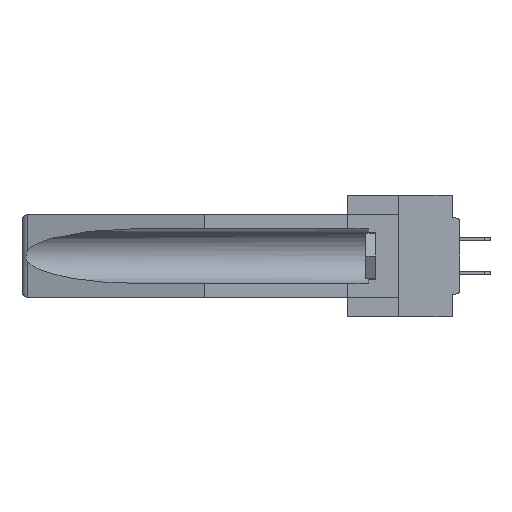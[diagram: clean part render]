
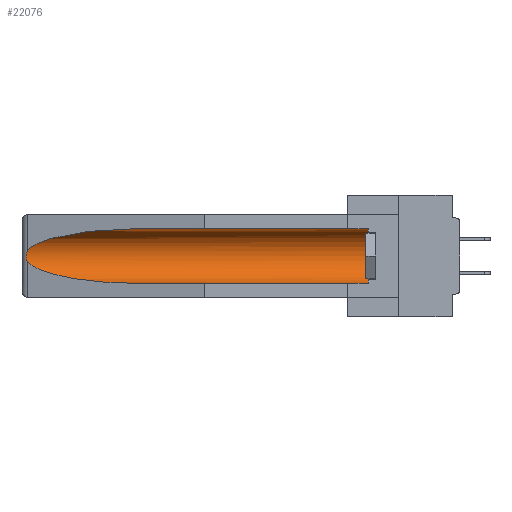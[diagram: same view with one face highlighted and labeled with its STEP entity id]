
A CAD part, left-side view. The second image highlights one B-rep face of the part: STEP entity #22076.
In plain terms, the highlighted cylindrical face has radius 2.857 mm (diameter 5.715 mm), a partial arc.
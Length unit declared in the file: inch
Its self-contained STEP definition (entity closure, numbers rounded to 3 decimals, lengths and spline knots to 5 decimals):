
#261 = CARTESIAN_POINT ( 'NONE',  ( 0.2673, 1.5327, -0.16383 ) ) ;
#477 = DIRECTION ( 'NONE',  ( 0., 0., 1. ) ) ;
#1191 = EDGE_CURVE ( 'NONE', #8287, #29350, #18271, .T. ) ;
#1553 = DIRECTION ( 'NONE',  ( 0., 1., 0. ) ) ;
#1906 = CYLINDRICAL_SURFACE ( 'NONE', #4686, 0.1125 ) ;
#2581 = VECTOR ( 'NONE', #31419, 39.37008 ) ;
#2783 = CARTESIAN_POINT ( 'NONE',  ( 0.26537, 1.52718, -0.14972 ) ) ;
#3278 = EDGE_CURVE ( 'NONE', #26897, #29350, #33648, .T. ) ;
#4251 = CARTESIAN_POINT ( 'NONE',  ( 0.155, 0.126, -0.1715 ) ) ;
#4686 = AXIS2_PLACEMENT_3D ( 'NONE', #19137, #5865, #477 ) ;
#5775 = CARTESIAN_POINT ( 'NONE',  ( 0.26537, 1.52718, -0.14972 ) ) ;
#5865 = DIRECTION ( 'NONE',  ( 0., 1., 0. ) ) ;
#5871 = LINE ( 'NONE', #21099, #2581 ) ;
#6681 = EDGE_LOOP ( 'NONE', ( #30616, #13603, #9948, #15802, #29697, #26227 ) ) ;
#6843 = EDGE_CURVE ( 'NONE', #8287, #15773, #15491, .T. ) ;
#7047 = CARTESIAN_POINT ( 'NONE',  ( 0.25451, 1.48313, -0.09465 ) ) ;
#8269 = CARTESIAN_POINT ( 'NONE',  ( 0.155, 1.07973, -0.284 ) ) ;
#8287 = VERTEX_POINT ( 'NONE', #11975 ) ;
#8763 = CARTESIAN_POINT ( 'NONE',  ( 0.26655, 1.53094, -0.18657 ) ) ;
#8972 = CARTESIAN_POINT ( 'NONE',  ( 0.155, 1.07973, -0.059 ) ) ;
#9255 = CARTESIAN_POINT ( 'NONE',  ( 0.26537, 1.52718, -0.14972 ) ) ;
#9948 = ORIENTED_EDGE ( 'NONE', *, *, #3278, .T. ) ;
#10777 = CARTESIAN_POINT ( 'NONE',  ( 0.2675, 1.53308, -0.17534 ) ) ;
#11446 = CARTESIAN_POINT ( 'NONE',  ( 0.155, 1.07973, -0.284 ) ) ;
#11547 = CARTESIAN_POINT ( 'NONE',  ( 0.26537, 1.52718, -0.19328 ) ) ;
#11863 = VERTEX_POINT ( 'NONE', #8972 ) ;
#11953 = CARTESIAN_POINT ( 'NONE',  ( 0.155, -0.30754, -0.284 ) ) ;
#11975 = CARTESIAN_POINT ( 'NONE',  ( 0.155, 0.126, -0.284 ) ) ;
#13603 = ORIENTED_EDGE ( 'NONE', *, *, #27464, .T. ) ;
#14019 = CARTESIAN_POINT ( 'NONE',  ( 0.21114, 1.30732, -0.284 ) ) ;
#14381 = EDGE_CURVE ( 'NONE', #11863, #25682, #33209, .T. ) ;
#15491 = CIRCLE ( 'NONE', #28461, 0.1125 ) ;
#15773 = VERTEX_POINT ( 'NONE', #25791 ) ;
#15802 = ORIENTED_EDGE ( 'NONE', *, *, #1191, .F. ) ;
#16107 = CARTESIAN_POINT ( 'NONE',  ( 0.2675, 1.53308, -0.16763 ) ) ;
#18271 = LINE ( 'NONE', #11953, #32357 ) ;
#19137 = CARTESIAN_POINT ( 'NONE',  ( 0.155, -0.30754, -0.1715 ) ) ;
#21099 = CARTESIAN_POINT ( 'NONE',  ( 0.155, -0.30754, -0.059 ) ) ;
#22053 = CARTESIAN_POINT ( 'NONE',  ( 0.26537, 1.52718, -0.19328 ) ) ;
#22076 = ADVANCED_FACE ( 'NONE', ( #30542 ), #1906, .F. ) ;
#22987 = CARTESIAN_POINT ( 'NONE',  ( 0.21114, 1.30732, -0.059 ) ) ;
#23305 = DIRECTION ( 'NONE',  ( 0., -1., 0. ) ) ;
#23872 = B_SPLINE_CURVE_WITH_KNOTS ( 'NONE', 3,
 ( #5775, #24029, #26701, #261, #16107, #10777, #29366, #8763, #27479, #11547 ),
 .UNSPECIFIED., .F., .F.,
 ( 4, 2, 2, 2, 4 ),
 ( 0., 0.00029, 0.00058, 0.00087, 0.00117 ),
 .UNSPECIFIED. ) ;
#24029 = CARTESIAN_POINT ( 'NONE',  ( 0.26597, 1.52961, -0.15275 ) ) ;
#24496 = CARTESIAN_POINT ( 'NONE',  ( 0.26537, 1.52718, -0.19328 ) ) ;
#24629 = EDGE_CURVE ( 'NONE', #15773, #11863, #5871, .T. ) ;
#25682 = VERTEX_POINT ( 'NONE', #2783 ) ;
#25791 = CARTESIAN_POINT ( 'NONE',  ( 0.155, 0.126, -0.059 ) ) ;
#26227 = ORIENTED_EDGE ( 'NONE', *, *, #24629, .T. ) ;
#26701 = CARTESIAN_POINT ( 'NONE',  ( 0.26654, 1.53092, -0.15636 ) ) ;
#26897 = VERTEX_POINT ( 'NONE', #24496 ) ;
#27464 = EDGE_CURVE ( 'NONE', #25682, #26897, #23872, .T. ) ;
#27479 = CARTESIAN_POINT ( 'NONE',  ( 0.26597, 1.5296, -0.19026 ) ) ;
#28461 = AXIS2_PLACEMENT_3D ( 'NONE', #4251, #23305, #28992 ) ;
#28992 = DIRECTION ( 'NONE',  ( 0., 0., 1. ) ) ;
#29350 = VERTEX_POINT ( 'NONE', #8269 ) ;
#29366 = CARTESIAN_POINT ( 'NONE',  ( 0.2673, 1.53269, -0.17917 ) ) ;
#29697 = ORIENTED_EDGE ( 'NONE', *, *, #6843, .T. ) ;
#30542 = FACE_OUTER_BOUND ( 'NONE', #6681, .T. ) ;
#30616 = ORIENTED_EDGE ( 'NONE', *, *, #14381, .T. ) ;
#31419 = DIRECTION ( 'NONE',  ( 0., 1., 0. ) ) ;
#32254 = CARTESIAN_POINT ( 'NONE',  ( 0.25451, 1.48313, -0.24835 ) ) ;
#32357 = VECTOR ( 'NONE', #1553, 39.37008 ) ;
#33209 =( BOUNDED_CURVE ( )  B_SPLINE_CURVE ( 3, ( #33545, #22987, #7047, #9255 ),
 .UNSPECIFIED., .F., .F. ) 
 B_SPLINE_CURVE_WITH_KNOTS ( ( 4, 4 ),
 ( 4.71239, 6.08839 ),
 .UNSPECIFIED. ) 
 CURVE ( )  GEOMETRIC_REPRESENTATION_ITEM ( )  RATIONAL_B_SPLINE_CURVE ( ( 1., 0.848, 0.848, 1. ) ) 
 REPRESENTATION_ITEM ( '' )  );
#33545 = CARTESIAN_POINT ( 'NONE',  ( 0.155, 1.07973, -0.059 ) ) ;
#33648 =( BOUNDED_CURVE ( )  B_SPLINE_CURVE ( 3, ( #22053, #32254, #14019, #11446 ),
 .UNSPECIFIED., .F., .F. ) 
 B_SPLINE_CURVE_WITH_KNOTS ( ( 4, 4 ),
 ( 0.1948, 1.5708 ),
 .UNSPECIFIED. ) 
 CURVE ( )  GEOMETRIC_REPRESENTATION_ITEM ( )  RATIONAL_B_SPLINE_CURVE ( ( 1., 0.848, 0.848, 1. ) ) 
 REPRESENTATION_ITEM ( '' )  );
